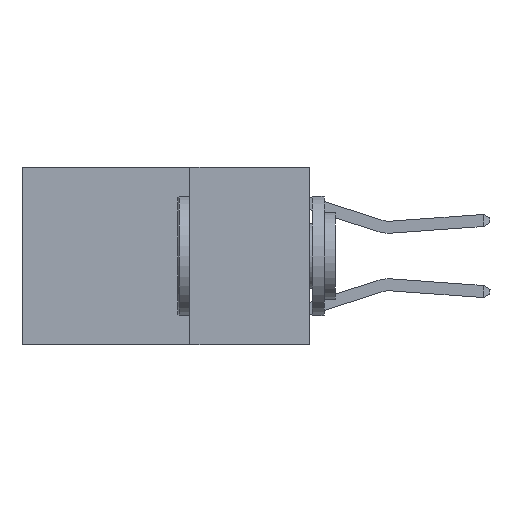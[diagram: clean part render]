
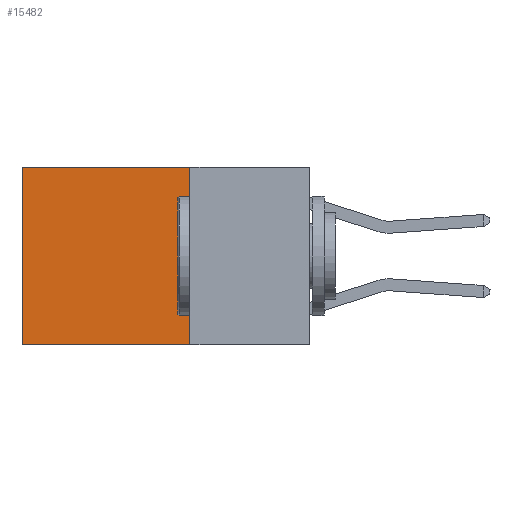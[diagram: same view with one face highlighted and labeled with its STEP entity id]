
A CAD part, left-side view. The second image highlights one B-rep face of the part: STEP entity #15482.
In plain terms, the highlighted planar face has unit normal (-1, 0, 0).
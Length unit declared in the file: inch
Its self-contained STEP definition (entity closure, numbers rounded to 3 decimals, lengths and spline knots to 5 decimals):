
#587 = EDGE_CURVE ( 'NONE', #17806, #15119, #15182, .T. ) ;
#2453 = LINE ( 'NONE', #8914, #10294 ) ;
#2594 = DIRECTION ( 'NONE',  ( 0., 0., -1. ) ) ;
#3148 = CARTESIAN_POINT ( 'NONE',  ( 0.2625, 0.25, -0.37 ) ) ;
#3577 = VECTOR ( 'NONE', #11684, 39.37008 ) ;
#7485 = VECTOR ( 'NONE', #23678, 39.37008 ) ;
#7639 = CARTESIAN_POINT ( 'NONE',  ( 0.2625, 0.25, 0. ) ) ;
#7704 = CARTESIAN_POINT ( 'NONE',  ( 0.2625, 0.25, -0.37 ) ) ;
#8071 = CARTESIAN_POINT ( 'NONE',  ( 0.2625, 0.6, -0.37 ) ) ;
#8499 = CARTESIAN_POINT ( 'NONE',  ( 0.2625, 0.25, 0. ) ) ;
#8914 = CARTESIAN_POINT ( 'NONE',  ( 0.2625, 0.6, 0. ) ) ;
#9682 = AXIS2_PLACEMENT_3D ( 'NONE', #7639, #20741, #22558 ) ;
#9758 = VECTOR ( 'NONE', #15801, 39.37008 ) ;
#10294 = VECTOR ( 'NONE', #2594, 39.37008 ) ;
#10927 = EDGE_LOOP ( 'NONE', ( #20400, #24125, #15384, #21379 ) ) ;
#11684 = DIRECTION ( 'NONE',  ( 0., 1., 0. ) ) ;
#11917 = CARTESIAN_POINT ( 'NONE',  ( 0.2625, 0.25, 0. ) ) ;
#13917 = LINE ( 'NONE', #3148, #3577 ) ;
#14651 = CARTESIAN_POINT ( 'NONE',  ( 0.2625, 0.6, 0. ) ) ;
#15119 = VERTEX_POINT ( 'NONE', #7704 ) ;
#15182 = LINE ( 'NONE', #8499, #7485 ) ;
#15384 = ORIENTED_EDGE ( 'NONE', *, *, #587, .F. ) ;
#15482 = ADVANCED_FACE ( 'NONE', ( #20890 ), #26720, .F. ) ;
#15801 = DIRECTION ( 'NONE',  ( 0., 1., 0. ) ) ;
#17806 = VERTEX_POINT ( 'NONE', #11917 ) ;
#19520 = EDGE_CURVE ( 'NONE', #17806, #22957, #23871, .T. ) ;
#19827 = CARTESIAN_POINT ( 'NONE',  ( 0.2625, 0.25, 0. ) ) ;
#20400 = ORIENTED_EDGE ( 'NONE', *, *, #21857, .T. ) ;
#20741 = DIRECTION ( 'NONE',  ( 1., 0., 0. ) ) ;
#20890 = FACE_OUTER_BOUND ( 'NONE', #10927, .T. ) ;
#21379 = ORIENTED_EDGE ( 'NONE', *, *, #19520, .T. ) ;
#21857 = EDGE_CURVE ( 'NONE', #22957, #24978, #2453, .T. ) ;
#21999 = EDGE_CURVE ( 'NONE', #15119, #24978, #13917, .T. ) ;
#22558 = DIRECTION ( 'NONE',  ( 0., 0., -1. ) ) ;
#22957 = VERTEX_POINT ( 'NONE', #14651 ) ;
#23678 = DIRECTION ( 'NONE',  ( 0., 0., -1. ) ) ;
#23871 = LINE ( 'NONE', #19827, #9758 ) ;
#24125 = ORIENTED_EDGE ( 'NONE', *, *, #21999, .F. ) ;
#24978 = VERTEX_POINT ( 'NONE', #8071 ) ;
#26720 = PLANE ( 'NONE',  #9682 ) ;
